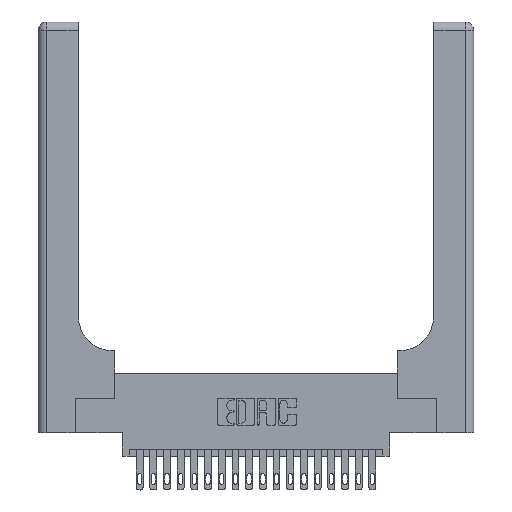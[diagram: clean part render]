
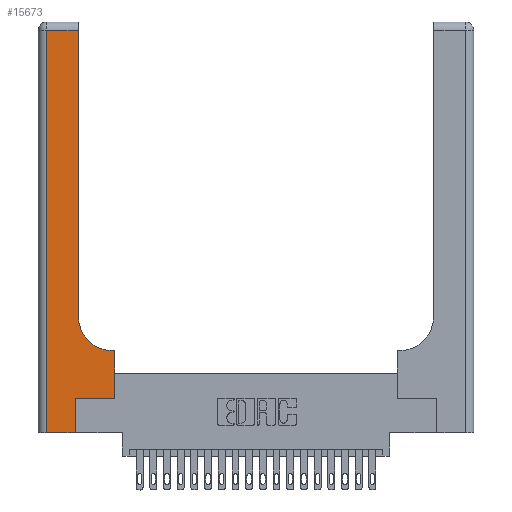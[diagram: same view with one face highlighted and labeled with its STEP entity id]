
A CAD part, top view. The second image highlights one B-rep face of the part: STEP entity #15673.
In plain terms, the highlighted planar face has unit normal (0, 0, 1).
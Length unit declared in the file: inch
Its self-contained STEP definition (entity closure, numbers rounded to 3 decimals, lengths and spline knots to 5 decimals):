
#166 = EDGE_CURVE ( 'NONE', #6151, #1061, #19270, .T. ) ;
#399 = VECTOR ( 'NONE', #20472, 39.37008 ) ;
#844 = AXIS2_PLACEMENT_3D ( 'NONE', #2908, #20516, #16930 ) ;
#974 = CARTESIAN_POINT ( 'NONE',  ( 0.5585, 0.6, 0.37 ) ) ;
#1061 = VERTEX_POINT ( 'NONE', #14078 ) ;
#1557 = DIRECTION ( 'NONE',  ( 1., 0., 0. ) ) ;
#2908 = CARTESIAN_POINT ( 'NONE',  ( 0., 3., 0.37 ) ) ;
#3247 = CIRCLE ( 'NONE', #4682, 0.25 ) ;
#4116 = VECTOR ( 'NONE', #21142, 39.37008 ) ;
#4682 = AXIS2_PLACEMENT_3D ( 'NONE', #7644, #7563, #14530 ) ;
#4695 = VERTEX_POINT ( 'NONE', #15776 ) ;
#4700 = LINE ( 'NONE', #7144, #14532 ) ;
#5890 = LINE ( 'NONE', #13709, #14066 ) ;
#5899 = VERTEX_POINT ( 'NONE', #9974 ) ;
#6151 = VERTEX_POINT ( 'NONE', #16898 ) ;
#6351 = DIRECTION ( 'NONE',  ( 0., 1., 0. ) ) ;
#6618 = EDGE_CURVE ( 'NONE', #4695, #15942, #8187, .T. ) ;
#7144 = CARTESIAN_POINT ( 'NONE',  ( 0.269, 0.25, 0.37 ) ) ;
#7165 = ORIENTED_EDGE ( 'NONE', *, *, #15236, .T. ) ;
#7226 = DIRECTION ( 'NONE',  ( -1., 0., 0. ) ) ;
#7563 = DIRECTION ( 'NONE',  ( 0., 0., -1. ) ) ;
#7644 = CARTESIAN_POINT ( 'NONE',  ( 0.5415, 0.85, 0.37 ) ) ;
#8187 = LINE ( 'NONE', #18461, #16029 ) ;
#8216 = EDGE_LOOP ( 'NONE', ( #20733, #11217, #20682, #22210, #15489, #7165, #13115, #18285, #21213 ) ) ;
#8424 = EDGE_CURVE ( 'NONE', #18164, #17687, #14903, .T. ) ;
#9209 = CARTESIAN_POINT ( 'NONE',  ( 0., 2.94, 0.37 ) ) ;
#9974 = CARTESIAN_POINT ( 'NONE',  ( 0.2915, 0.85, 0.37 ) ) ;
#10492 = EDGE_CURVE ( 'NONE', #17687, #13815, #19131, .T. ) ;
#10862 = CARTESIAN_POINT ( 'NONE',  ( 0.269, 0.25, 0.37 ) ) ;
#11217 = ORIENTED_EDGE ( 'NONE', *, *, #21415, .T. ) ;
#11568 = CARTESIAN_POINT ( 'NONE',  ( 0.2915, 2.94, 0.37 ) ) ;
#11576 = DIRECTION ( 'NONE',  ( 0., 1., 0. ) ) ;
#12686 = VECTOR ( 'NONE', #7226, 39.37008 ) ;
#13115 = ORIENTED_EDGE ( 'NONE', *, *, #8424, .T. ) ;
#13709 = CARTESIAN_POINT ( 'NONE',  ( 0., 0., 0.37 ) ) ;
#13815 = VERTEX_POINT ( 'NONE', #22188 ) ;
#14066 = VECTOR ( 'NONE', #1557, 39.37008 ) ;
#14078 = CARTESIAN_POINT ( 'NONE',  ( 0.06, 0., 0.37 ) ) ;
#14147 = CARTESIAN_POINT ( 'NONE',  ( 0.2915, 0.6, 0.37 ) ) ;
#14282 = FACE_OUTER_BOUND ( 'NONE', #8216, .T. ) ;
#14505 = EDGE_CURVE ( 'NONE', #1061, #4695, #5890, .T. ) ;
#14530 = DIRECTION ( 'NONE',  ( 1., 0., 0. ) ) ;
#14532 = VECTOR ( 'NONE', #15814, 39.37008 ) ;
#14903 = LINE ( 'NONE', #18705, #399 ) ;
#15236 = EDGE_CURVE ( 'NONE', #15942, #18164, #4700, .T. ) ;
#15398 = LINE ( 'NONE', #21902, #18655 ) ;
#15489 = ORIENTED_EDGE ( 'NONE', *, *, #6618, .T. ) ;
#15571 = EDGE_CURVE ( 'NONE', #5899, #15616, #15398, .T. ) ;
#15616 = VERTEX_POINT ( 'NONE', #11568 ) ;
#15673 = ADVANCED_FACE ( 'NONE', ( #14282 ), #20437, .F. ) ;
#15776 = CARTESIAN_POINT ( 'NONE',  ( 0.269, 0., 0.37 ) ) ;
#15814 = DIRECTION ( 'NONE',  ( 1., 0., 0. ) ) ;
#15942 = VERTEX_POINT ( 'NONE', #10862 ) ;
#16029 = VECTOR ( 'NONE', #11576, 39.37008 ) ;
#16898 = CARTESIAN_POINT ( 'NONE',  ( 0.06, 2.94, 0.37 ) ) ;
#16930 = DIRECTION ( 'NONE',  ( -1., 0., 0. ) ) ;
#17216 = DIRECTION ( 'NONE',  ( 0., -1., 0. ) ) ;
#17687 = VERTEX_POINT ( 'NONE', #974 ) ;
#18164 = VERTEX_POINT ( 'NONE', #18205 ) ;
#18205 = CARTESIAN_POINT ( 'NONE',  ( 0.5585, 0.25, 0.37 ) ) ;
#18285 = ORIENTED_EDGE ( 'NONE', *, *, #10492, .T. ) ;
#18461 = CARTESIAN_POINT ( 'NONE',  ( 0.269, 0., 0.37 ) ) ;
#18655 = VECTOR ( 'NONE', #6351, 39.37008 ) ;
#18705 = CARTESIAN_POINT ( 'NONE',  ( 0.5585, 0.25, 0.37 ) ) ;
#18729 = CARTESIAN_POINT ( 'NONE',  ( 0.06, 3., 0.37 ) ) ;
#19116 = EDGE_CURVE ( 'NONE', #13815, #5899, #3247, .T. ) ;
#19131 = LINE ( 'NONE', #14147, #4116 ) ;
#19270 = LINE ( 'NONE', #18729, #20910 ) ;
#20437 = PLANE ( 'NONE',  #844 ) ;
#20472 = DIRECTION ( 'NONE',  ( 0., 1., 0. ) ) ;
#20516 = DIRECTION ( 'NONE',  ( 0., 0., -1. ) ) ;
#20682 = ORIENTED_EDGE ( 'NONE', *, *, #166, .T. ) ;
#20733 = ORIENTED_EDGE ( 'NONE', *, *, #15571, .T. ) ;
#20910 = VECTOR ( 'NONE', #17216, 39.37008 ) ;
#21142 = DIRECTION ( 'NONE',  ( -1., 0., 0. ) ) ;
#21213 = ORIENTED_EDGE ( 'NONE', *, *, #19116, .T. ) ;
#21415 = EDGE_CURVE ( 'NONE', #15616, #6151, #22242, .T. ) ;
#21902 = CARTESIAN_POINT ( 'NONE',  ( 0.2915, 3., 0.37 ) ) ;
#22188 = CARTESIAN_POINT ( 'NONE',  ( 0.5415, 0.6, 0.37 ) ) ;
#22210 = ORIENTED_EDGE ( 'NONE', *, *, #14505, .T. ) ;
#22242 = LINE ( 'NONE', #9209, #12686 ) ;
